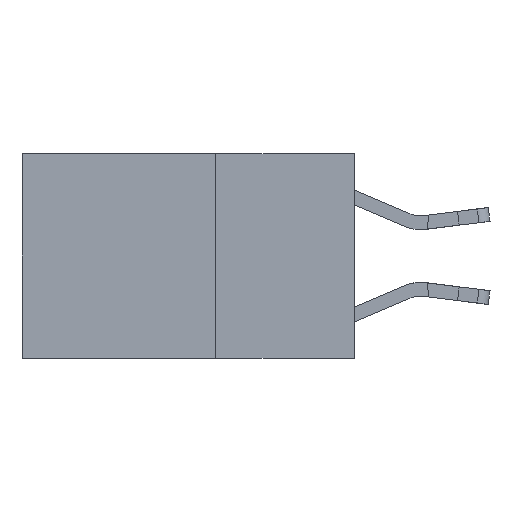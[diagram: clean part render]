
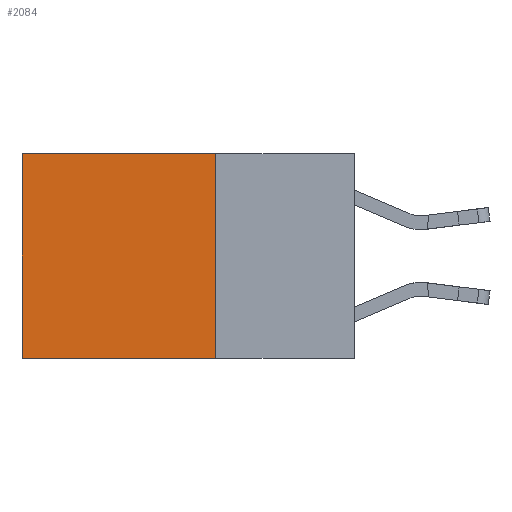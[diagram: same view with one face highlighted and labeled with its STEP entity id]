
A CAD part, left-side view. The second image highlights one B-rep face of the part: STEP entity #2084.
In plain terms, the highlighted planar face has unit normal (-1, 0, 0).
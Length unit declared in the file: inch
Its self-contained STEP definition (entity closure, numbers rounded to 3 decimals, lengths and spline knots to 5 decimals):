
#515 = CARTESIAN_POINT ( 'NONE',  ( 0.2625, 0.6, 0. ) ) ;
#710 = CARTESIAN_POINT ( 'NONE',  ( 0.2625, 0.25, 0. ) ) ;
#1311 = CARTESIAN_POINT ( 'NONE',  ( 0.2625, 0.25, -0.37 ) ) ;
#1442 = CARTESIAN_POINT ( 'NONE',  ( 0.2625, 0.25, 0. ) ) ;
#2084 = ADVANCED_FACE ( 'NONE', ( #7927 ), #10287, .F. ) ;
#2467 = CARTESIAN_POINT ( 'NONE',  ( 0.2625, 0.6, 0. ) ) ;
#2524 = DIRECTION ( 'NONE',  ( 0., 1., 0. ) ) ;
#2629 = VECTOR ( 'NONE', #10829, 39.37008 ) ;
#3484 = CARTESIAN_POINT ( 'NONE',  ( 0.2625, 0.25, 0. ) ) ;
#4569 = VERTEX_POINT ( 'NONE', #12206 ) ;
#4640 = VERTEX_POINT ( 'NONE', #710 ) ;
#5489 = LINE ( 'NONE', #1311, #11417 ) ;
#5924 = DIRECTION ( 'NONE',  ( 0., 0., -1. ) ) ;
#6040 = ORIENTED_EDGE ( 'NONE', *, *, #10086, .F. ) ;
#6403 = ORIENTED_EDGE ( 'NONE', *, *, #10134, .T. ) ;
#6963 = VERTEX_POINT ( 'NONE', #515 ) ;
#7213 = ORIENTED_EDGE ( 'NONE', *, *, #10516, .F. ) ;
#7563 = LINE ( 'NONE', #11930, #2629 ) ;
#7791 = DIRECTION ( 'NONE',  ( 1., 0., 0. ) ) ;
#7927 = FACE_OUTER_BOUND ( 'NONE', #8147, .T. ) ;
#8080 = VERTEX_POINT ( 'NONE', #9369 ) ;
#8147 = EDGE_LOOP ( 'NONE', ( #12279, #6040, #7213, #6403 ) ) ;
#8395 = VECTOR ( 'NONE', #5924, 39.37008 ) ;
#8426 = EDGE_CURVE ( 'NONE', #6963, #4569, #13251, .T. ) ;
#9369 = CARTESIAN_POINT ( 'NONE',  ( 0.2625, 0.25, -0.37 ) ) ;
#10086 = EDGE_CURVE ( 'NONE', #8080, #4569, #5489, .T. ) ;
#10134 = EDGE_CURVE ( 'NONE', #4640, #6963, #12160, .T. ) ;
#10287 = PLANE ( 'NONE',  #13451 ) ;
#10516 = EDGE_CURVE ( 'NONE', #4640, #8080, #7563, .T. ) ;
#10829 = DIRECTION ( 'NONE',  ( 0., 0., -1. ) ) ;
#11417 = VECTOR ( 'NONE', #2524, 39.37008 ) ;
#11930 = CARTESIAN_POINT ( 'NONE',  ( 0.2625, 0.25, 0. ) ) ;
#12160 = LINE ( 'NONE', #1442, #12370 ) ;
#12206 = CARTESIAN_POINT ( 'NONE',  ( 0.2625, 0.6, -0.37 ) ) ;
#12279 = ORIENTED_EDGE ( 'NONE', *, *, #8426, .T. ) ;
#12313 = DIRECTION ( 'NONE',  ( 0., 0., -1. ) ) ;
#12370 = VECTOR ( 'NONE', #13532, 39.37008 ) ;
#13251 = LINE ( 'NONE', #2467, #8395 ) ;
#13451 = AXIS2_PLACEMENT_3D ( 'NONE', #3484, #7791, #12313 ) ;
#13532 = DIRECTION ( 'NONE',  ( 0., 1., 0. ) ) ;
